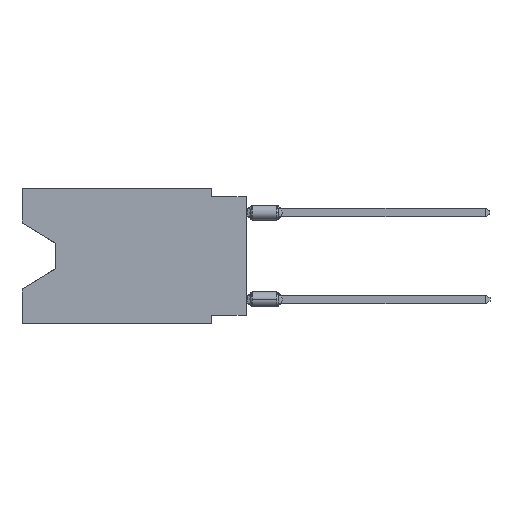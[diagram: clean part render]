
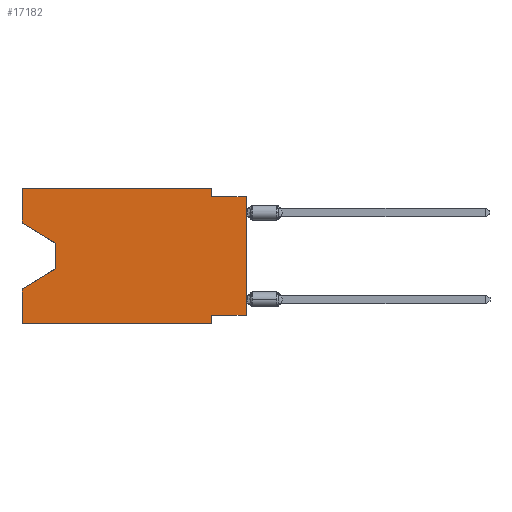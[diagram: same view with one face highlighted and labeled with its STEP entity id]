
A CAD part, left-side view. The second image highlights one B-rep face of the part: STEP entity #17182.
In plain terms, the highlighted planar face has unit normal (-1, 0, 0).
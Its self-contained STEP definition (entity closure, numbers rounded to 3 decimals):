
#289 = CARTESIAN_POINT ( 'NONE',  ( 0., 16.383, 0. ) ) ;
#337 = CARTESIAN_POINT ( 'NONE',  ( 0., 16.383, 0. ) ) ;
#392 = DIRECTION ( 'NONE',  ( 0., 1., 0. ) ) ;
#647 = DIRECTION ( 'NONE',  ( 0., -0.855, -0.519 ) ) ;
#1375 = LINE ( 'NONE', #9693, #25823 ) ;
#2381 = VECTOR ( 'NONE', #12497, 1000. ) ;
#2831 = CARTESIAN_POINT ( 'NONE',  ( 0., 16.383, -9.906 ) ) ;
#3412 = ORIENTED_EDGE ( 'NONE', *, *, #9418, .F. ) ;
#4111 = EDGE_CURVE ( 'NONE', #24942, #25929, #8532, .T. ) ;
#4265 = CARTESIAN_POINT ( 'NONE',  ( 0., 2.54, 0. ) ) ;
#4400 = LINE ( 'NONE', #4265, #13901 ) ;
#4573 = CARTESIAN_POINT ( 'NONE',  ( 0., 16.383, 0. ) ) ;
#4604 = ORIENTED_EDGE ( 'NONE', *, *, #7435, .F. ) ;
#6318 = CARTESIAN_POINT ( 'NONE',  ( 0., 0., -0.635 ) ) ;
#6571 = DIRECTION ( 'NONE',  ( 1., 0., 0. ) ) ;
#6635 = ORIENTED_EDGE ( 'NONE', *, *, #7879, .F. ) ;
#6755 = LINE ( 'NONE', #337, #17489 ) ;
#6886 = VECTOR ( 'NONE', #23558, 1000. ) ;
#6964 = EDGE_CURVE ( 'NONE', #22025, #24942, #14857, .T. ) ;
#7174 = EDGE_LOOP ( 'NONE', ( #22263, #18506, #23382, #10371, #24811, #3412, #25485, #22407, #15301, #6635, #10746, #4604 ) ) ;
#7435 = EDGE_CURVE ( 'NONE', #22025, #18500, #19047, .T. ) ;
#7571 = EDGE_CURVE ( 'NONE', #19841, #26936, #11520, .T. ) ;
#7636 = EDGE_CURVE ( 'NONE', #25929, #19215, #15757, .T. ) ;
#7879 = EDGE_CURVE ( 'NONE', #23072, #19365, #4400, .T. ) ;
#8477 = CARTESIAN_POINT ( 'NONE',  ( 0., 2.54, -9.906 ) ) ;
#8532 = LINE ( 'NONE', #14290, #2381 ) ;
#9117 = CARTESIAN_POINT ( 'NONE',  ( 0., 2.54, -9.271 ) ) ;
#9418 = EDGE_CURVE ( 'NONE', #24670, #17245, #1375, .T. ) ;
#9465 = VECTOR ( 'NONE', #647, 1000. ) ;
#9693 = CARTESIAN_POINT ( 'NONE',  ( 0., 2.54, -9.906 ) ) ;
#10189 = CARTESIAN_POINT ( 'NONE',  ( 0., 16.383, -7.36 ) ) ;
#10371 = ORIENTED_EDGE ( 'NONE', *, *, #22771, .F. ) ;
#10387 = DIRECTION ( 'NONE',  ( 0., 0., -1. ) ) ;
#10746 = ORIENTED_EDGE ( 'NONE', *, *, #14223, .F. ) ;
#10785 = DIRECTION ( 'NONE',  ( 0., 0., -1. ) ) ;
#10810 = VECTOR ( 'NONE', #10836, 1000. ) ;
#10836 = DIRECTION ( 'NONE',  ( 0., 0., 1. ) ) ;
#11108 = CARTESIAN_POINT ( 'NONE',  ( 0., 0., -9.271 ) ) ;
#11213 = CARTESIAN_POINT ( 'NONE',  ( 0., 13.97, -4.013 ) ) ;
#11520 = LINE ( 'NONE', #17819, #6886 ) ;
#12316 = FACE_OUTER_BOUND ( 'NONE', #7174, .T. ) ;
#12497 = DIRECTION ( 'NONE',  ( 0., 0., -1. ) ) ;
#12650 = LINE ( 'NONE', #18941, #25909 ) ;
#13615 = LINE ( 'NONE', #21947, #21346 ) ;
#13646 = CARTESIAN_POINT ( 'NONE',  ( 0., 13.97, -5.893 ) ) ;
#13677 = CARTESIAN_POINT ( 'NONE',  ( 0., 16.383, 0. ) ) ;
#13901 = VECTOR ( 'NONE', #10387, 1000. ) ;
#14223 = EDGE_CURVE ( 'NONE', #18500, #23072, #6755, .T. ) ;
#14290 = CARTESIAN_POINT ( 'NONE',  ( 0., 13.97, -4.013 ) ) ;
#14336 = LINE ( 'NONE', #19097, #26688 ) ;
#14857 = LINE ( 'NONE', #21541, #9465 ) ;
#14892 = LINE ( 'NONE', #25128, #17657 ) ;
#15257 = EDGE_CURVE ( 'NONE', #24471, #17245, #13615, .T. ) ;
#15301 = ORIENTED_EDGE ( 'NONE', *, *, #21989, .F. ) ;
#15757 = LINE ( 'NONE', #24096, #24345 ) ;
#16498 = CARTESIAN_POINT ( 'NONE',  ( 0., 16.383, -2.546 ) ) ;
#17085 = DIRECTION ( 'NONE',  ( 0., 0., 1. ) ) ;
#17182 = ADVANCED_FACE ( 'NONE', ( #12316 ), #21180, .F. ) ;
#17245 = VERTEX_POINT ( 'NONE', #8477 ) ;
#17416 = DIRECTION ( 'NONE',  ( 0., -1., 0. ) ) ;
#17489 = VECTOR ( 'NONE', #17416, 1000. ) ;
#17611 = EDGE_CURVE ( 'NONE', #19841, #24670, #14336, .T. ) ;
#17657 = VECTOR ( 'NONE', #17085, 1000. ) ;
#17819 = CARTESIAN_POINT ( 'NONE',  ( 0., 0., 0. ) ) ;
#18500 = VERTEX_POINT ( 'NONE', #13677 ) ;
#18506 = ORIENTED_EDGE ( 'NONE', *, *, #4111, .T. ) ;
#18669 = DIRECTION ( 'NONE',  ( 0., -1., 0. ) ) ;
#18941 = CARTESIAN_POINT ( 'NONE',  ( 0., 0., -0.635 ) ) ;
#19047 = LINE ( 'NONE', #4573, #10810 ) ;
#19097 = CARTESIAN_POINT ( 'NONE',  ( 0., 0., -9.271 ) ) ;
#19215 = VERTEX_POINT ( 'NONE', #10189 ) ;
#19340 = CARTESIAN_POINT ( 'NONE',  ( 0., 2.54, -0.635 ) ) ;
#19365 = VERTEX_POINT ( 'NONE', #19340 ) ;
#19841 = VERTEX_POINT ( 'NONE', #11108 ) ;
#19887 = DIRECTION ( 'NONE',  ( 0., -1., 0. ) ) ;
#20854 = CARTESIAN_POINT ( 'NONE',  ( 0., 2.54, 0. ) ) ;
#20911 = AXIS2_PLACEMENT_3D ( 'NONE', #289, #6571, #10785 ) ;
#21180 = PLANE ( 'NONE',  #20911 ) ;
#21346 = VECTOR ( 'NONE', #19887, 1000. ) ;
#21503 = DIRECTION ( 'NONE',  ( 0., 0.855, -0.519 ) ) ;
#21541 = CARTESIAN_POINT ( 'NONE',  ( 0., 16.383, -2.546 ) ) ;
#21947 = CARTESIAN_POINT ( 'NONE',  ( 0., 16.383, -9.906 ) ) ;
#21989 = EDGE_CURVE ( 'NONE', #19365, #26936, #12650, .T. ) ;
#22025 = VERTEX_POINT ( 'NONE', #16498 ) ;
#22263 = ORIENTED_EDGE ( 'NONE', *, *, #6964, .T. ) ;
#22407 = ORIENTED_EDGE ( 'NONE', *, *, #7571, .T. ) ;
#22771 = EDGE_CURVE ( 'NONE', #24471, #19215, #14892, .T. ) ;
#23072 = VERTEX_POINT ( 'NONE', #20854 ) ;
#23382 = ORIENTED_EDGE ( 'NONE', *, *, #7636, .T. ) ;
#23558 = DIRECTION ( 'NONE',  ( 0., 0., 1. ) ) ;
#24096 = CARTESIAN_POINT ( 'NONE',  ( 0., 13.97, -5.893 ) ) ;
#24345 = VECTOR ( 'NONE', #21503, 1000. ) ;
#24471 = VERTEX_POINT ( 'NONE', #2831 ) ;
#24670 = VERTEX_POINT ( 'NONE', #9117 ) ;
#24811 = ORIENTED_EDGE ( 'NONE', *, *, #15257, .T. ) ;
#24942 = VERTEX_POINT ( 'NONE', #11213 ) ;
#25128 = CARTESIAN_POINT ( 'NONE',  ( 0., 16.383, 0. ) ) ;
#25485 = ORIENTED_EDGE ( 'NONE', *, *, #17611, .F. ) ;
#25823 = VECTOR ( 'NONE', #26233, 1000. ) ;
#25909 = VECTOR ( 'NONE', #18669, 1000. ) ;
#25929 = VERTEX_POINT ( 'NONE', #13646 ) ;
#26233 = DIRECTION ( 'NONE',  ( 0., 0., -1. ) ) ;
#26688 = VECTOR ( 'NONE', #392, 1000. ) ;
#26936 = VERTEX_POINT ( 'NONE', #6318 ) ;
